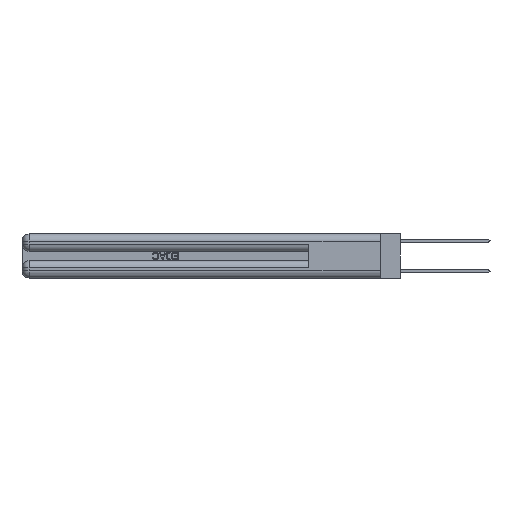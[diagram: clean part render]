
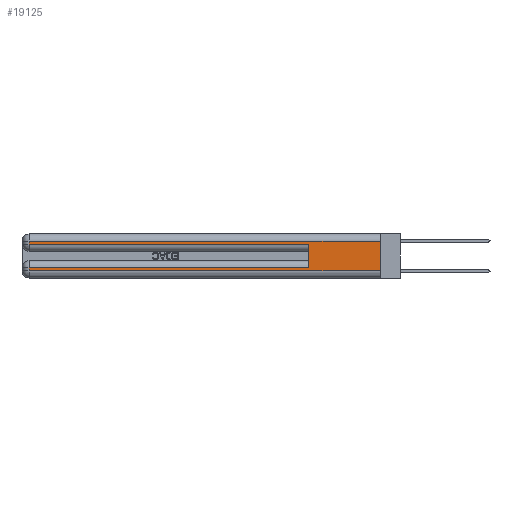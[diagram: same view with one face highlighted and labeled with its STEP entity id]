
A CAD part, left-side view. The second image highlights one B-rep face of the part: STEP entity #19125.
In plain terms, the highlighted planar face has unit normal (-1, 0, 0).
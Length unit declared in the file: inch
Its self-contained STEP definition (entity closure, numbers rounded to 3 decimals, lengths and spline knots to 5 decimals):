
#968 = CARTESIAN_POINT ( 'NONE',  ( 0., 0., 0.37 ) ) ;
#1073 = EDGE_CURVE ( 'NONE', #25915, #2200, #23078, .T. ) ;
#1593 = CARTESIAN_POINT ( 'NONE',  ( 0., 0., 0.085 ) ) ;
#1693 = VECTOR ( 'NONE', #26384, 39.37008 ) ;
#1748 = VECTOR ( 'NONE', #17722, 39.37008 ) ;
#2053 = DIRECTION ( 'NONE',  ( 0., 0., -1. ) ) ;
#2200 = VERTEX_POINT ( 'NONE', #8133 ) ;
#2729 = VERTEX_POINT ( 'NONE', #12984 ) ;
#3234 = VECTOR ( 'NONE', #25478, 39.37008 ) ;
#3863 = VECTOR ( 'NONE', #10700, 39.37008 ) ;
#5159 = ORIENTED_EDGE ( 'NONE', *, *, #30693, .F. ) ;
#5170 = VERTEX_POINT ( 'NONE', #23367 ) ;
#5480 = CARTESIAN_POINT ( 'NONE',  ( 0., 0., 0.06 ) ) ;
#6736 = ORIENTED_EDGE ( 'NONE', *, *, #23675, .T. ) ;
#6806 = EDGE_CURVE ( 'NONE', #23284, #5170, #12267, .T. ) ;
#6909 = LINE ( 'NONE', #9763, #9145 ) ;
#7290 = LINE ( 'NONE', #1593, #15622 ) ;
#7333 = CARTESIAN_POINT ( 'NONE',  ( 0., 2.94, 0.37 ) ) ;
#7665 = CARTESIAN_POINT ( 'NONE',  ( 0., 0., 0.31 ) ) ;
#8133 = CARTESIAN_POINT ( 'NONE',  ( 0., 0.6, 0.285 ) ) ;
#8189 = DIRECTION ( 'NONE',  ( 0., 0., -1. ) ) ;
#9145 = VECTOR ( 'NONE', #20347, 39.37008 ) ;
#9763 = CARTESIAN_POINT ( 'NONE',  ( 0., 2.94, 0.37 ) ) ;
#10240 = DIRECTION ( 'NONE',  ( 0., 1., 0. ) ) ;
#10700 = DIRECTION ( 'NONE',  ( 0., -1., 0. ) ) ;
#12267 = LINE ( 'NONE', #20489, #30390 ) ;
#12319 = ORIENTED_EDGE ( 'NONE', *, *, #23092, .T. ) ;
#12809 = CARTESIAN_POINT ( 'NONE',  ( 0., 0., 0.06 ) ) ;
#12984 = CARTESIAN_POINT ( 'NONE',  ( 0., 2.94, 0.06 ) ) ;
#13354 = CARTESIAN_POINT ( 'NONE',  ( 0., 0., 0.285 ) ) ;
#14243 = VECTOR ( 'NONE', #8189, 39.37008 ) ;
#15375 = EDGE_CURVE ( 'NONE', #2729, #24690, #23464, .T. ) ;
#15622 = VECTOR ( 'NONE', #22575, 39.37008 ) ;
#17354 = DIRECTION ( 'NONE',  ( 1., 0., 0. ) ) ;
#17425 = AXIS2_PLACEMENT_3D ( 'NONE', #33140, #17354, #2053 ) ;
#17519 = FACE_OUTER_BOUND ( 'NONE', #30597, .T. ) ;
#17574 = VERTEX_POINT ( 'NONE', #18995 ) ;
#17722 = DIRECTION ( 'NONE',  ( 0., -1., 0. ) ) ;
#18995 = CARTESIAN_POINT ( 'NONE',  ( 0., 2.94, 0.085 ) ) ;
#19125 = ADVANCED_FACE ( 'NONE', ( #17519 ), #20366, .F. ) ;
#20347 = DIRECTION ( 'NONE',  ( 0., 0., -1. ) ) ;
#20366 = PLANE ( 'NONE',  #17425 ) ;
#20489 = CARTESIAN_POINT ( 'NONE',  ( 0., 0., 0.31 ) ) ;
#20957 = EDGE_CURVE ( 'NONE', #5170, #25915, #6909, .T. ) ;
#21285 = LINE ( 'NONE', #968, #14243 ) ;
#21837 = LINE ( 'NONE', #32104, #1693 ) ;
#22219 = ORIENTED_EDGE ( 'NONE', *, *, #6806, .T. ) ;
#22455 = LINE ( 'NONE', #7333, #3234 ) ;
#22575 = DIRECTION ( 'NONE',  ( 0., 1., 0. ) ) ;
#23078 = LINE ( 'NONE', #13354, #1748 ) ;
#23092 = EDGE_CURVE ( 'NONE', #17574, #2729, #22455, .T. ) ;
#23284 = VERTEX_POINT ( 'NONE', #7665 ) ;
#23367 = CARTESIAN_POINT ( 'NONE',  ( 0., 2.94, 0.31 ) ) ;
#23464 = LINE ( 'NONE', #5480, #3863 ) ;
#23675 = EDGE_CURVE ( 'NONE', #25835, #17574, #7290, .T. ) ;
#24142 = ORIENTED_EDGE ( 'NONE', *, *, #1073, .T. ) ;
#24261 = ORIENTED_EDGE ( 'NONE', *, *, #20957, .T. ) ;
#24690 = VERTEX_POINT ( 'NONE', #12809 ) ;
#24907 = EDGE_CURVE ( 'NONE', #25835, #2200, #21837, .T. ) ;
#25478 = DIRECTION ( 'NONE',  ( 0., 0., -1. ) ) ;
#25835 = VERTEX_POINT ( 'NONE', #33139 ) ;
#25915 = VERTEX_POINT ( 'NONE', #26229 ) ;
#26229 = CARTESIAN_POINT ( 'NONE',  ( 0., 2.94, 0.285 ) ) ;
#26384 = DIRECTION ( 'NONE',  ( 0., 0., 1. ) ) ;
#29524 = ORIENTED_EDGE ( 'NONE', *, *, #15375, .T. ) ;
#30390 = VECTOR ( 'NONE', #10240, 39.37008 ) ;
#30597 = EDGE_LOOP ( 'NONE', ( #5159, #22219, #24261, #24142, #32445, #6736, #12319, #29524 ) ) ;
#30693 = EDGE_CURVE ( 'NONE', #23284, #24690, #21285, .T. ) ;
#32104 = CARTESIAN_POINT ( 'NONE',  ( 0., 0.6, 0.145 ) ) ;
#32445 = ORIENTED_EDGE ( 'NONE', *, *, #24907, .F. ) ;
#33139 = CARTESIAN_POINT ( 'NONE',  ( 0., 0.6, 0.085 ) ) ;
#33140 = CARTESIAN_POINT ( 'NONE',  ( 0., 0., 0.37 ) ) ;
